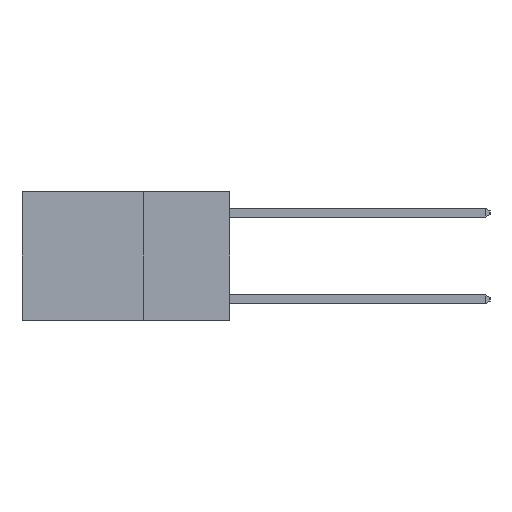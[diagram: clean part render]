
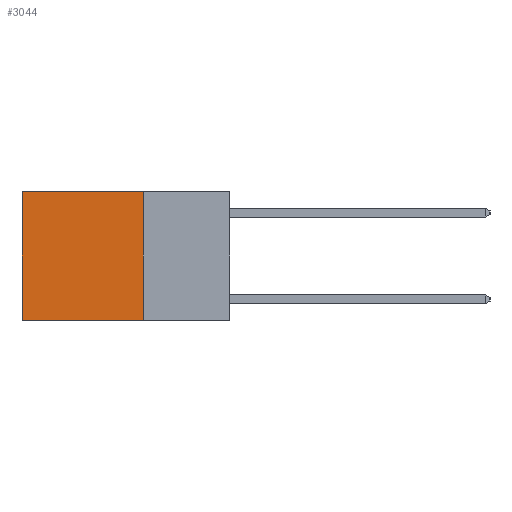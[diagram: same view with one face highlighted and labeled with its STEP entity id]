
A CAD part, left-side view. The second image highlights one B-rep face of the part: STEP entity #3044.
In plain terms, the highlighted planar face has unit normal (-1, 0, 0).
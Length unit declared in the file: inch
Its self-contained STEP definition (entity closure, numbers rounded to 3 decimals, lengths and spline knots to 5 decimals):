
#334 = ORIENTED_EDGE ( 'NONE', *, *, #6400, .T. ) ;
#588 = LINE ( 'NONE', #9056, #12128 ) ;
#954 = CARTESIAN_POINT ( 'NONE',  ( 0.2625, 0.25, 0. ) ) ;
#1309 = EDGE_CURVE ( 'NONE', #11142, #15586, #10986, .T. ) ;
#2044 = EDGE_CURVE ( 'NONE', #15586, #13673, #3937, .T. ) ;
#2522 = DIRECTION ( 'NONE',  ( 0., 1., 0. ) ) ;
#2823 = DIRECTION ( 'NONE',  ( 0., 1., 0. ) ) ;
#3044 = ADVANCED_FACE ( 'NONE', ( #11642 ), #15567, .F. ) ;
#3733 = LINE ( 'NONE', #10108, #9554 ) ;
#3815 = VERTEX_POINT ( 'NONE', #7399 ) ;
#3937 = LINE ( 'NONE', #13929, #7865 ) ;
#4032 = AXIS2_PLACEMENT_3D ( 'NONE', #15489, #6793, #14212 ) ;
#5231 = DIRECTION ( 'NONE',  ( 0., 0., -1. ) ) ;
#5808 = EDGE_LOOP ( 'NONE', ( #9137, #6332, #10067, #334 ) ) ;
#6332 = ORIENTED_EDGE ( 'NONE', *, *, #2044, .F. ) ;
#6400 = EDGE_CURVE ( 'NONE', #11142, #3815, #3733, .T. ) ;
#6777 = CARTESIAN_POINT ( 'NONE',  ( 0.2625, 0.25, -0.37 ) ) ;
#6793 = DIRECTION ( 'NONE',  ( 1., 0., 0. ) ) ;
#7399 = CARTESIAN_POINT ( 'NONE',  ( 0.2625, 0.6, 0. ) ) ;
#7865 = VECTOR ( 'NONE', #2823, 39.37008 ) ;
#8810 = EDGE_CURVE ( 'NONE', #3815, #13673, #588, .T. ) ;
#9056 = CARTESIAN_POINT ( 'NONE',  ( 0.2625, 0.6, 0. ) ) ;
#9137 = ORIENTED_EDGE ( 'NONE', *, *, #8810, .T. ) ;
#9554 = VECTOR ( 'NONE', #2522, 39.37008 ) ;
#10067 = ORIENTED_EDGE ( 'NONE', *, *, #1309, .F. ) ;
#10108 = CARTESIAN_POINT ( 'NONE',  ( 0.2625, 0.25, 0. ) ) ;
#10986 = LINE ( 'NONE', #12040, #15255 ) ;
#11142 = VERTEX_POINT ( 'NONE', #954 ) ;
#11642 = FACE_OUTER_BOUND ( 'NONE', #5808, .T. ) ;
#12040 = CARTESIAN_POINT ( 'NONE',  ( 0.2625, 0.25, 0. ) ) ;
#12128 = VECTOR ( 'NONE', #5231, 39.37008 ) ;
#13673 = VERTEX_POINT ( 'NONE', #14983 ) ;
#13929 = CARTESIAN_POINT ( 'NONE',  ( 0.2625, 0.25, -0.37 ) ) ;
#14212 = DIRECTION ( 'NONE',  ( 0., 0., -1. ) ) ;
#14983 = CARTESIAN_POINT ( 'NONE',  ( 0.2625, 0.6, -0.37 ) ) ;
#15255 = VECTOR ( 'NONE', #15895, 39.37008 ) ;
#15489 = CARTESIAN_POINT ( 'NONE',  ( 0.2625, 0.25, 0. ) ) ;
#15567 = PLANE ( 'NONE',  #4032 ) ;
#15586 = VERTEX_POINT ( 'NONE', #6777 ) ;
#15895 = DIRECTION ( 'NONE',  ( 0., 0., -1. ) ) ;
